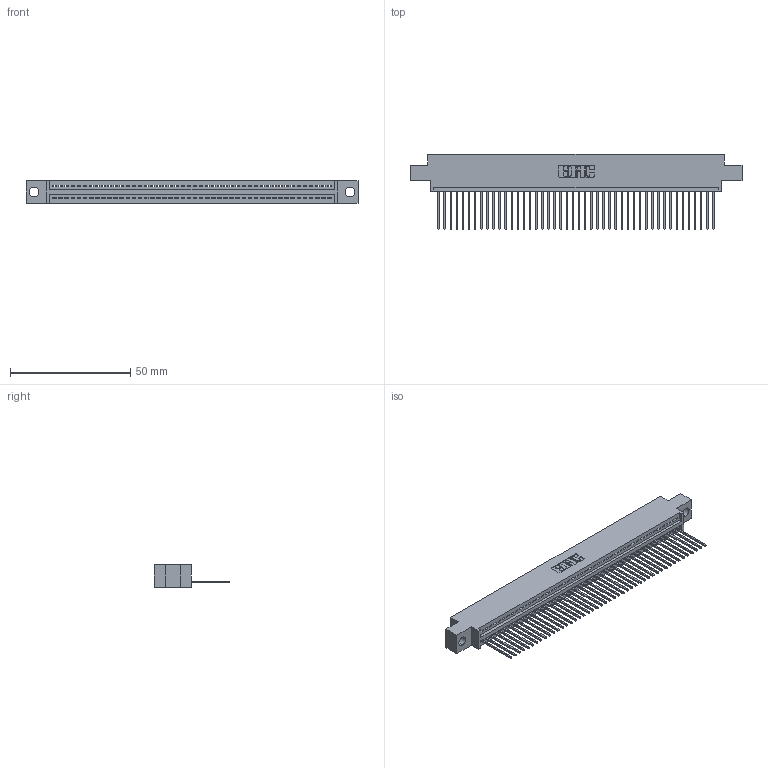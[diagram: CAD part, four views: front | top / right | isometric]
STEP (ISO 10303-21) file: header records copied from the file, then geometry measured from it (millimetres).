
FILE_DESCRIPTION (( 'STEP AP203' ), '1' );
FILE_NAME ('395-046-542-604.STEP', '2021-05-31T15:13:34', ( '' ), ( '' ), 'SwSTEP 2.0', 'SolidWorks 2020', '' );
FILE_SCHEMA (( 'CONFIG_CONTROL_DESIGN' ));
Length unit declared in the file: inch
Products named in the file (3): 345 Part_0.170 Offset - 0.156 Dia-TI; 395-046-542-604; 345-292-001_345-293-142
Assembly tree (47 placements, depth 2):
  395-046-542-604
    345 Part_0.170 Offset - 0.156 Dia-TI
    345-292-001_345-293-142  x46
Bounding box: 138.05 x 31.29 x 9.4 mm (x, y, z)
Volume: 13027.8 mm3; surface area: 17983.4 mm2
Topology: 47 solids, 47 shells, 2812 faces, 8485 edges, 5594 vertices
Faces by surface type: plane 1938, cylinder 874
Entity records: 34651 total; most frequent: CARTESIAN_POINT 6012, ORIENTED_EDGE 5990, DIRECTION 5243, EDGE_CURVE 2995, LINE 2679, VECTOR 2679, VERTEX_POINT 1994, AXIS2_PLACEMENT_3D 1282
